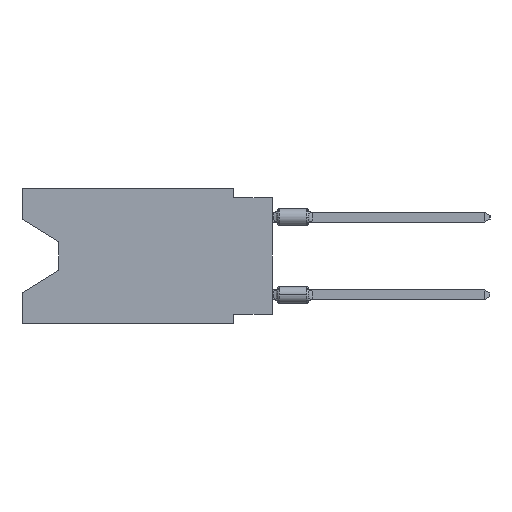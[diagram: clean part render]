
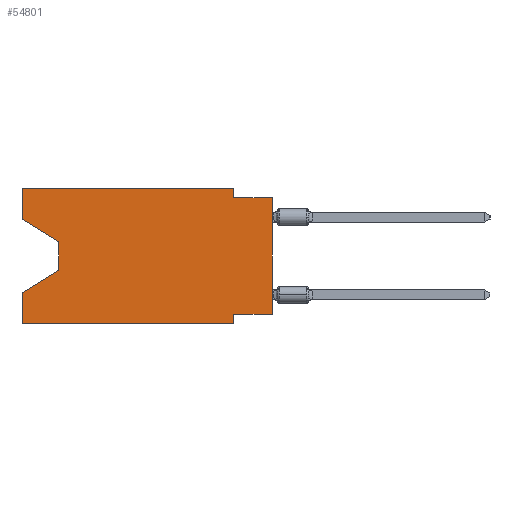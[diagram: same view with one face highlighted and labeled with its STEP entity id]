
A CAD part, left-side view. The second image highlights one B-rep face of the part: STEP entity #54801.
In plain terms, the highlighted planar face has unit normal (-1, 0, 0).
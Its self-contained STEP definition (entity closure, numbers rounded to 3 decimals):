
#95 = DIRECTION ( 'NONE',  ( 0., 1., 0. ) ) ;
#592 = VECTOR ( 'NONE', #53388, 1000. ) ;
#1469 = EDGE_CURVE ( 'NONE', #40279, #48526, #20001, .T. ) ;
#3732 = DIRECTION ( 'NONE',  ( 0., -1., 0. ) ) ;
#4012 = CARTESIAN_POINT ( 'NONE',  ( 0., 2.54, -8.89 ) ) ;
#4965 = LINE ( 'NONE', #44599, #8247 ) ;
#5526 = CARTESIAN_POINT ( 'NONE',  ( 0., 2.54, 0. ) ) ;
#5610 = LINE ( 'NONE', #53444, #22355 ) ;
#7311 = DIRECTION ( 'NONE',  ( 0., -0.855, -0.519 ) ) ;
#7490 = CARTESIAN_POINT ( 'NONE',  ( 0., 16.383, 0. ) ) ;
#7731 = ORIENTED_EDGE ( 'NONE', *, *, #61398, .T. ) ;
#7805 = PLANE ( 'NONE',  #48611 ) ;
#8247 = VECTOR ( 'NONE', #95, 1000. ) ;
#10257 = VECTOR ( 'NONE', #40617, 1000. ) ;
#10690 = CARTESIAN_POINT ( 'NONE',  ( 0., 0., -8.255 ) ) ;
#11009 = VECTOR ( 'NONE', #46807, 1000. ) ;
#11203 = VERTEX_POINT ( 'NONE', #12624 ) ;
#11407 = ORIENTED_EDGE ( 'NONE', *, *, #51357, .F. ) ;
#11758 = CARTESIAN_POINT ( 'NONE',  ( 0., 13.97, -3.505 ) ) ;
#12624 = CARTESIAN_POINT ( 'NONE',  ( 0., 16.383, -6.852 ) ) ;
#12634 = CARTESIAN_POINT ( 'NONE',  ( 0., 2.54, 0. ) ) ;
#13233 = CARTESIAN_POINT ( 'NONE',  ( 0., 2.54, -0.635 ) ) ;
#14627 = VERTEX_POINT ( 'NONE', #17019 ) ;
#15427 = EDGE_LOOP ( 'NONE', ( #7731, #15726, #55836, #21306, #56807, #22530, #11407, #44944, #37369, #45871, #61872, #57623 ) ) ;
#15726 = ORIENTED_EDGE ( 'NONE', *, *, #52757, .T. ) ;
#16296 = VECTOR ( 'NONE', #52729, 1000. ) ;
#17019 = CARTESIAN_POINT ( 'NONE',  ( 0., 2.54, -8.89 ) ) ;
#18349 = VERTEX_POINT ( 'NONE', #63167 ) ;
#20001 = LINE ( 'NONE', #63830, #21451 ) ;
#21306 = ORIENTED_EDGE ( 'NONE', *, *, #47391, .F. ) ;
#21451 = VECTOR ( 'NONE', #39814, 1000. ) ;
#22355 = VECTOR ( 'NONE', #38511, 1000. ) ;
#22530 = ORIENTED_EDGE ( 'NONE', *, *, #34348, .F. ) ;
#26841 = CARTESIAN_POINT ( 'NONE',  ( 0., 13.97, -5.385 ) ) ;
#26987 = CARTESIAN_POINT ( 'NONE',  ( 0., 16.383, 0. ) ) ;
#27195 = EDGE_CURVE ( 'NONE', #48526, #37553, #48240, .T. ) ;
#29005 = LINE ( 'NONE', #58876, #57088 ) ;
#29669 = EDGE_CURVE ( 'NONE', #37553, #41930, #62619, .T. ) ;
#29964 = DIRECTION ( 'NONE',  ( 0., 0., 1. ) ) ;
#30800 = EDGE_CURVE ( 'NONE', #41930, #44368, #45178, .T. ) ;
#31263 = LINE ( 'NONE', #11758, #55715 ) ;
#31438 = FACE_OUTER_BOUND ( 'NONE', #15427, .T. ) ;
#32925 = CARTESIAN_POINT ( 'NONE',  ( 0., 0., -0.635 ) ) ;
#33470 = CARTESIAN_POINT ( 'NONE',  ( 0., 0., -0.635 ) ) ;
#33588 = LINE ( 'NONE', #4012, #592 ) ;
#34348 = EDGE_CURVE ( 'NONE', #44951, #14627, #33588, .T. ) ;
#36727 = DIRECTION ( 'NONE',  ( 0., 0., -1. ) ) ;
#37128 = VERTEX_POINT ( 'NONE', #48573 ) ;
#37369 = ORIENTED_EDGE ( 'NONE', *, *, #30800, .F. ) ;
#37374 = DIRECTION ( 'NONE',  ( 1., 0., 0. ) ) ;
#37553 = VERTEX_POINT ( 'NONE', #5526 ) ;
#38497 = CARTESIAN_POINT ( 'NONE',  ( 0., 16.383, 0. ) ) ;
#38511 = DIRECTION ( 'NONE',  ( 0., -1., 0. ) ) ;
#39814 = DIRECTION ( 'NONE',  ( 0., 0., 1. ) ) ;
#39988 = CARTESIAN_POINT ( 'NONE',  ( 0., 13.97, -5.385 ) ) ;
#40279 = VERTEX_POINT ( 'NONE', #57790 ) ;
#40617 = DIRECTION ( 'NONE',  ( 0., 0.855, -0.519 ) ) ;
#41616 = LINE ( 'NONE', #7490, #11009 ) ;
#41930 = VERTEX_POINT ( 'NONE', #13233 ) ;
#42263 = CARTESIAN_POINT ( 'NONE',  ( 0., 16.383, 0. ) ) ;
#44368 = VERTEX_POINT ( 'NONE', #33470 ) ;
#44599 = CARTESIAN_POINT ( 'NONE',  ( 0., 0., -8.255 ) ) ;
#44944 = ORIENTED_EDGE ( 'NONE', *, *, #56298, .T. ) ;
#44951 = VERTEX_POINT ( 'NONE', #62121 ) ;
#45178 = LINE ( 'NONE', #32925, #16296 ) ;
#45871 = ORIENTED_EDGE ( 'NONE', *, *, #29669, .F. ) ;
#46111 = LINE ( 'NONE', #39988, #10257 ) ;
#46507 = EDGE_CURVE ( 'NONE', #37128, #14627, #5610, .T. ) ;
#46807 = DIRECTION ( 'NONE',  ( 0., 0., 1. ) ) ;
#47011 = VECTOR ( 'NONE', #7311, 1000. ) ;
#47391 = EDGE_CURVE ( 'NONE', #37128, #11203, #41616, .T. ) ;
#48089 = VECTOR ( 'NONE', #3732, 1000. ) ;
#48240 = LINE ( 'NONE', #38497, #48089 ) ;
#48526 = VERTEX_POINT ( 'NONE', #42263 ) ;
#48573 = CARTESIAN_POINT ( 'NONE',  ( 0., 16.383, -8.89 ) ) ;
#48611 = AXIS2_PLACEMENT_3D ( 'NONE', #26987, #37374, #36727 ) ;
#50101 = EDGE_CURVE ( 'NONE', #56888, #11203, #46111, .T. ) ;
#51357 = EDGE_CURVE ( 'NONE', #55115, #44951, #4965, .T. ) ;
#51388 = DIRECTION ( 'NONE',  ( 0., 0., -1. ) ) ;
#52729 = DIRECTION ( 'NONE',  ( 0., -1., 0. ) ) ;
#52757 = EDGE_CURVE ( 'NONE', #18349, #56888, #31263, .T. ) ;
#53388 = DIRECTION ( 'NONE',  ( 0., 0., -1. ) ) ;
#53444 = CARTESIAN_POINT ( 'NONE',  ( 0., 16.383, -8.89 ) ) ;
#54801 = ADVANCED_FACE ( 'NONE', ( #31438 ), #7805, .F. ) ;
#55115 = VERTEX_POINT ( 'NONE', #10690 ) ;
#55715 = VECTOR ( 'NONE', #51388, 1000. ) ;
#55836 = ORIENTED_EDGE ( 'NONE', *, *, #50101, .T. ) ;
#56298 = EDGE_CURVE ( 'NONE', #55115, #44368, #29005, .T. ) ;
#56807 = ORIENTED_EDGE ( 'NONE', *, *, #46507, .T. ) ;
#56888 = VERTEX_POINT ( 'NONE', #26841 ) ;
#57005 = CARTESIAN_POINT ( 'NONE',  ( 0., 16.383, -2.038 ) ) ;
#57088 = VECTOR ( 'NONE', #29964, 1000. ) ;
#57133 = DIRECTION ( 'NONE',  ( 0., 0., -1. ) ) ;
#57623 = ORIENTED_EDGE ( 'NONE', *, *, #1469, .F. ) ;
#57790 = CARTESIAN_POINT ( 'NONE',  ( 0., 16.383, -2.038 ) ) ;
#58876 = CARTESIAN_POINT ( 'NONE',  ( 0., 0., 0. ) ) ;
#61398 = EDGE_CURVE ( 'NONE', #40279, #18349, #61861, .T. ) ;
#61861 = LINE ( 'NONE', #57005, #47011 ) ;
#61872 = ORIENTED_EDGE ( 'NONE', *, *, #27195, .F. ) ;
#62121 = CARTESIAN_POINT ( 'NONE',  ( 0., 2.54, -8.255 ) ) ;
#62619 = LINE ( 'NONE', #12634, #62803 ) ;
#62803 = VECTOR ( 'NONE', #57133, 1000. ) ;
#63167 = CARTESIAN_POINT ( 'NONE',  ( 0., 13.97, -3.505 ) ) ;
#63830 = CARTESIAN_POINT ( 'NONE',  ( 0., 16.383, 0. ) ) ;
